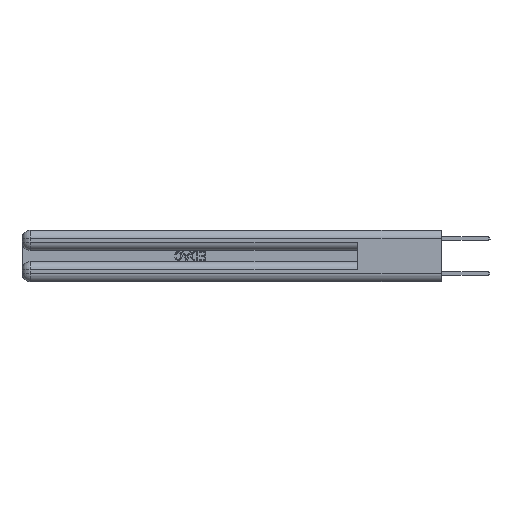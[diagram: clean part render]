
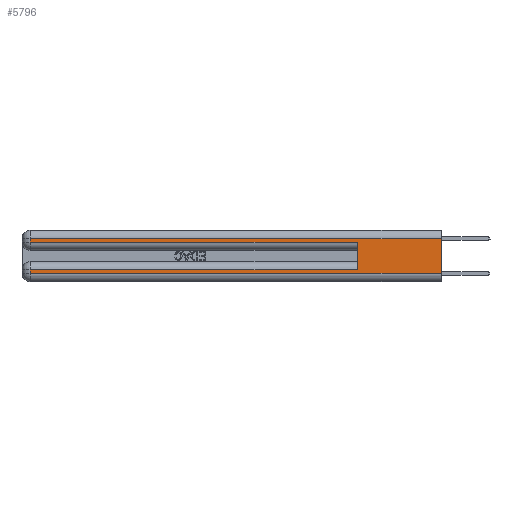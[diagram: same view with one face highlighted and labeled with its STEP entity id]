
A CAD part, left-side view. The second image highlights one B-rep face of the part: STEP entity #5796.
In plain terms, the highlighted planar face has unit normal (-1, 0, 0).
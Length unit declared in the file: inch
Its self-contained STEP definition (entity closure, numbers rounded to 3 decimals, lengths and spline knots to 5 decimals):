
#200 = LINE ( 'NONE', #4896, #11393 ) ;
#1601 = ORIENTED_EDGE ( 'NONE', *, *, #3617, .T. ) ;
#2283 = VECTOR ( 'NONE', #20443, 39.37008 ) ;
#2295 = CARTESIAN_POINT ( 'NONE',  ( 0., 0.6, 0.085 ) ) ;
#3570 = VECTOR ( 'NONE', #13241, 39.37008 ) ;
#3617 = EDGE_CURVE ( 'NONE', #24265, #9073, #22672, .T. ) ;
#4401 = ORIENTED_EDGE ( 'NONE', *, *, #13288, .T. ) ;
#4802 = VECTOR ( 'NONE', #26416, 39.37008 ) ;
#4896 = CARTESIAN_POINT ( 'NONE',  ( 0., 0., 0.085 ) ) ;
#5090 = CARTESIAN_POINT ( 'NONE',  ( 0., 0., 0.06 ) ) ;
#5304 = PLANE ( 'NONE',  #17832 ) ;
#5446 = LINE ( 'NONE', #6751, #12851 ) ;
#5796 = ADVANCED_FACE ( 'NONE', ( #18635 ), #5304, .F. ) ;
#5887 = CARTESIAN_POINT ( 'NONE',  ( 0., 2.94, 0.31 ) ) ;
#6175 = VERTEX_POINT ( 'NONE', #15968 ) ;
#6321 = EDGE_CURVE ( 'NONE', #23704, #6625, #8411, .T. ) ;
#6625 = VERTEX_POINT ( 'NONE', #26434 ) ;
#6751 = CARTESIAN_POINT ( 'NONE',  ( 0., 0.6, 0.145 ) ) ;
#8368 = DIRECTION ( 'NONE',  ( 0., 0., -1. ) ) ;
#8411 = LINE ( 'NONE', #21986, #18267 ) ;
#8590 = ORIENTED_EDGE ( 'NONE', *, *, #6321, .T. ) ;
#9073 = VERTEX_POINT ( 'NONE', #5090 ) ;
#9385 = ORIENTED_EDGE ( 'NONE', *, *, #28791, .T. ) ;
#9820 = DIRECTION ( 'NONE',  ( 0., 0., -1. ) ) ;
#10723 = CARTESIAN_POINT ( 'NONE',  ( 0., 0., 0.06 ) ) ;
#11006 = CARTESIAN_POINT ( 'NONE',  ( 0., 0., 0.37 ) ) ;
#11094 = VECTOR ( 'NONE', #8368, 39.37008 ) ;
#11393 = VECTOR ( 'NONE', #16359, 39.37008 ) ;
#11985 = CARTESIAN_POINT ( 'NONE',  ( 0., 0.6, 0.285 ) ) ;
#12176 = EDGE_CURVE ( 'NONE', #26833, #6175, #200, .T. ) ;
#12562 = EDGE_LOOP ( 'NONE', ( #16316, #19299, #8590, #4401, #23480, #18540, #9385, #1601 ) ) ;
#12851 = VECTOR ( 'NONE', #13229, 39.37008 ) ;
#13162 = DIRECTION ( 'NONE',  ( 0., -1., 0. ) ) ;
#13229 = DIRECTION ( 'NONE',  ( 0., 0., 1. ) ) ;
#13241 = DIRECTION ( 'NONE',  ( 0., 0., -1. ) ) ;
#13288 = EDGE_CURVE ( 'NONE', #6625, #15730, #20584, .T. ) ;
#13292 = CARTESIAN_POINT ( 'NONE',  ( 0., 0., 0.31 ) ) ;
#14127 = DIRECTION ( 'NONE',  ( 1., 0., 0. ) ) ;
#14154 = LINE ( 'NONE', #18201, #2283 ) ;
#15011 = EDGE_CURVE ( 'NONE', #23508, #23704, #14154, .T. ) ;
#15730 = VERTEX_POINT ( 'NONE', #11985 ) ;
#15968 = CARTESIAN_POINT ( 'NONE',  ( 0., 2.94, 0.085 ) ) ;
#16316 = ORIENTED_EDGE ( 'NONE', *, *, #27650, .F. ) ;
#16359 = DIRECTION ( 'NONE',  ( 0., 1., 0. ) ) ;
#17832 = AXIS2_PLACEMENT_3D ( 'NONE', #20998, #14127, #9820 ) ;
#18201 = CARTESIAN_POINT ( 'NONE',  ( 0., 0., 0.31 ) ) ;
#18267 = VECTOR ( 'NONE', #24420, 39.37008 ) ;
#18540 = ORIENTED_EDGE ( 'NONE', *, *, #12176, .T. ) ;
#18635 = FACE_OUTER_BOUND ( 'NONE', #12562, .T. ) ;
#19299 = ORIENTED_EDGE ( 'NONE', *, *, #15011, .T. ) ;
#19852 = CARTESIAN_POINT ( 'NONE',  ( 0., 0., 0.285 ) ) ;
#20443 = DIRECTION ( 'NONE',  ( 0., 1., 0. ) ) ;
#20584 = LINE ( 'NONE', #19852, #21282 ) ;
#20712 = EDGE_CURVE ( 'NONE', #26833, #15730, #5446, .T. ) ;
#20998 = CARTESIAN_POINT ( 'NONE',  ( 0., 0., 0.37 ) ) ;
#21282 = VECTOR ( 'NONE', #13162, 39.37008 ) ;
#21620 = CARTESIAN_POINT ( 'NONE',  ( 0., 2.94, 0.37 ) ) ;
#21986 = CARTESIAN_POINT ( 'NONE',  ( 0., 2.94, 0.37 ) ) ;
#22641 = LINE ( 'NONE', #21620, #11094 ) ;
#22672 = LINE ( 'NONE', #10723, #4802 ) ;
#23480 = ORIENTED_EDGE ( 'NONE', *, *, #20712, .F. ) ;
#23508 = VERTEX_POINT ( 'NONE', #13292 ) ;
#23704 = VERTEX_POINT ( 'NONE', #5887 ) ;
#23964 = CARTESIAN_POINT ( 'NONE',  ( 0., 2.94, 0.06 ) ) ;
#24265 = VERTEX_POINT ( 'NONE', #23964 ) ;
#24420 = DIRECTION ( 'NONE',  ( 0., 0., -1. ) ) ;
#24828 = LINE ( 'NONE', #11006, #3570 ) ;
#26416 = DIRECTION ( 'NONE',  ( 0., -1., 0. ) ) ;
#26434 = CARTESIAN_POINT ( 'NONE',  ( 0., 2.94, 0.285 ) ) ;
#26833 = VERTEX_POINT ( 'NONE', #2295 ) ;
#27650 = EDGE_CURVE ( 'NONE', #23508, #9073, #24828, .T. ) ;
#28791 = EDGE_CURVE ( 'NONE', #6175, #24265, #22641, .T. ) ;
